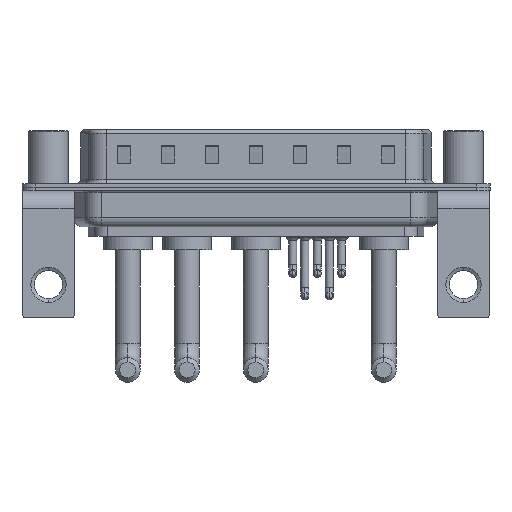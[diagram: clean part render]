
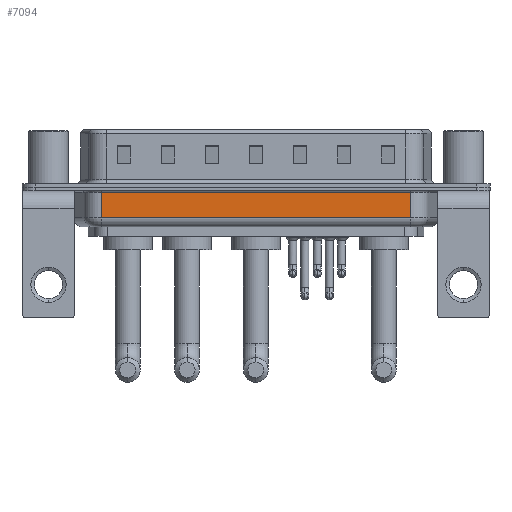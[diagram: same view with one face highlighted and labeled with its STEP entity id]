
A CAD part, front view. The second image highlights one B-rep face of the part: STEP entity #7094.
In plain terms, the highlighted planar face has unit normal (0, -1, 0).
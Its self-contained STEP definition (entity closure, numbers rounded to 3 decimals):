
#281 = LINE ( 'NONE', #8112, #9479 ) ;
#305 = VERTEX_POINT ( 'NONE', #15956 ) ;
#2170 = DIRECTION ( 'NONE',  ( -1., 0., 0. ) ) ;
#2449 = EDGE_CURVE ( 'NONE', #7814, #12454, #17818, .T. ) ;
#3382 = CARTESIAN_POINT ( 'NONE',  ( 6.006, -5.35, -4.5 ) ) ;
#3891 = LINE ( 'NONE', #3382, #11859 ) ;
#4176 = EDGE_CURVE ( 'NONE', #12454, #6623, #20977, .T. ) ;
#6552 = CARTESIAN_POINT ( 'NONE',  ( 6.006, -5.35, -4.5 ) ) ;
#6623 = VERTEX_POINT ( 'NONE', #12391 ) ;
#7094 = ADVANCED_FACE ( 'NONE', ( #16173 ), #23857, .F. ) ;
#7814 = VERTEX_POINT ( 'NONE', #23512 ) ;
#8098 = CARTESIAN_POINT ( 'NONE',  ( 6.006, -5.35, -3.5 ) ) ;
#8112 = CARTESIAN_POINT ( 'NONE',  ( 6.006, -5.35, -0.65 ) ) ;
#8239 = ORIENTED_EDGE ( 'NONE', *, *, #16033, .T. ) ;
#9479 = VECTOR ( 'NONE', #2170, 1000. ) ;
#11594 = DIRECTION ( 'NONE',  ( 0., 0., 1. ) ) ;
#11859 = VECTOR ( 'NONE', #11594, 1000. ) ;
#12391 = CARTESIAN_POINT ( 'NONE',  ( 41.044, -5.35, -0.65 ) ) ;
#12454 = VERTEX_POINT ( 'NONE', #23452 ) ;
#13429 = ORIENTED_EDGE ( 'NONE', *, *, #4176, .T. ) ;
#13961 = ORIENTED_EDGE ( 'NONE', *, *, #14266, .F. ) ;
#14266 = EDGE_CURVE ( 'NONE', #7814, #305, #3891, .T. ) ;
#14282 = DIRECTION ( 'NONE',  ( 0., 1., 0. ) ) ;
#14920 = DIRECTION ( 'NONE',  ( 0., 0., 1. ) ) ;
#15956 = CARTESIAN_POINT ( 'NONE',  ( 6.006, -5.35, -0.65 ) ) ;
#16021 = VECTOR ( 'NONE', #21493, 1000. ) ;
#16033 = EDGE_CURVE ( 'NONE', #6623, #305, #281, .T. ) ;
#16054 = VECTOR ( 'NONE', #14920, 1000. ) ;
#16173 = FACE_OUTER_BOUND ( 'NONE', #19157, .T. ) ;
#17785 = AXIS2_PLACEMENT_3D ( 'NONE', #6552, #14282, #21968 ) ;
#17818 = LINE ( 'NONE', #8098, #16021 ) ;
#19157 = EDGE_LOOP ( 'NONE', ( #13961, #19229, #13429, #8239 ) ) ;
#19229 = ORIENTED_EDGE ( 'NONE', *, *, #2449, .T. ) ;
#20977 = LINE ( 'NONE', #22990, #16054 ) ;
#21493 = DIRECTION ( 'NONE',  ( 1., 0., 0. ) ) ;
#21968 = DIRECTION ( 'NONE',  ( 0., 0., 1. ) ) ;
#22990 = CARTESIAN_POINT ( 'NONE',  ( 41.044, -5.35, -4.5 ) ) ;
#23452 = CARTESIAN_POINT ( 'NONE',  ( 41.044, -5.35, -3.5 ) ) ;
#23512 = CARTESIAN_POINT ( 'NONE',  ( 6.006, -5.35, -3.5 ) ) ;
#23857 = PLANE ( 'NONE',  #17785 ) ;
